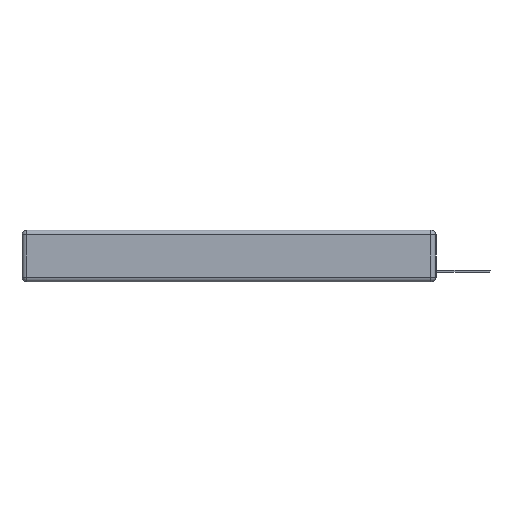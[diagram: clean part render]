
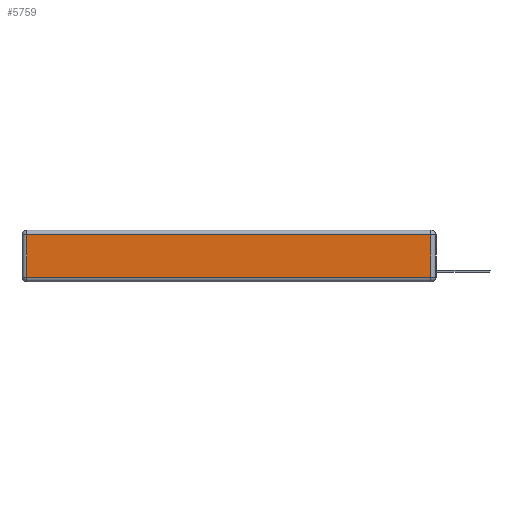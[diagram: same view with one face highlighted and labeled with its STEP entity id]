
A CAD part, left-side view. The second image highlights one B-rep face of the part: STEP entity #5759.
In plain terms, the highlighted planar face has unit normal (-1, 0, 0).
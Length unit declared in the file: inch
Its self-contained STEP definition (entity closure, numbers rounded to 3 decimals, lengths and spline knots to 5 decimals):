
#363 = CARTESIAN_POINT ( 'NONE',  ( 0., 0.03, -0.343 ) ) ;
#465 = EDGE_CURVE ( 'NONE', #4299, #11582, #4855, .T. ) ;
#637 = AXIS2_PLACEMENT_3D ( 'NONE', #4353, #4548, #9961 ) ;
#735 = PLANE ( 'NONE',  #637 ) ;
#736 = ORIENTED_EDGE ( 'NONE', *, *, #11382, .T. ) ;
#1600 = LINE ( 'NONE', #8040, #1606 ) ;
#1606 = VECTOR ( 'NONE', #5298, 39.37008 ) ;
#2235 = LINE ( 'NONE', #363, #11024 ) ;
#2990 = CARTESIAN_POINT ( 'NONE',  ( 0., 0.03, -0.03 ) ) ;
#4062 = EDGE_LOOP ( 'NONE', ( #9951, #736, #7886, #4384 ) ) ;
#4299 = VERTEX_POINT ( 'NONE', #2990 ) ;
#4353 = CARTESIAN_POINT ( 'NONE',  ( 0., 0., -0.343 ) ) ;
#4384 = ORIENTED_EDGE ( 'NONE', *, *, #9934, .T. ) ;
#4548 = DIRECTION ( 'NONE',  ( -1., 0., 0. ) ) ;
#4557 = EDGE_CURVE ( 'NONE', #6209, #8768, #1600, .T. ) ;
#4819 = VECTOR ( 'NONE', #6607, 39.37008 ) ;
#4855 = LINE ( 'NONE', #8523, #7484 ) ;
#5298 = DIRECTION ( 'NONE',  ( 0., -1., 0. ) ) ;
#5411 = CARTESIAN_POINT ( 'NONE',  ( 0., 2.72, -0.313 ) ) ;
#5759 = ADVANCED_FACE ( 'NONE', ( #6425 ), #735, .T. ) ;
#6209 = VERTEX_POINT ( 'NONE', #5411 ) ;
#6425 = FACE_OUTER_BOUND ( 'NONE', #4062, .T. ) ;
#6535 = CARTESIAN_POINT ( 'NONE',  ( 0., 2.72, -0.03 ) ) ;
#6602 = DIRECTION ( 'NONE',  ( 0., 1., 0. ) ) ;
#6607 = DIRECTION ( 'NONE',  ( 0., 0., -1. ) ) ;
#7484 = VECTOR ( 'NONE', #6602, 39.37008 ) ;
#7528 = LINE ( 'NONE', #11335, #4819 ) ;
#7886 = ORIENTED_EDGE ( 'NONE', *, *, #465, .T. ) ;
#8040 = CARTESIAN_POINT ( 'NONE',  ( 0., 0., -0.313 ) ) ;
#8265 = DIRECTION ( 'NONE',  ( 0., 0., 1. ) ) ;
#8523 = CARTESIAN_POINT ( 'NONE',  ( 0., 2.75, -0.03 ) ) ;
#8768 = VERTEX_POINT ( 'NONE', #10067 ) ;
#9934 = EDGE_CURVE ( 'NONE', #11582, #6209, #7528, .T. ) ;
#9951 = ORIENTED_EDGE ( 'NONE', *, *, #4557, .T. ) ;
#9961 = DIRECTION ( 'NONE',  ( 0., 0., 1. ) ) ;
#10067 = CARTESIAN_POINT ( 'NONE',  ( 0., 0.03, -0.313 ) ) ;
#11024 = VECTOR ( 'NONE', #8265, 39.37008 ) ;
#11335 = CARTESIAN_POINT ( 'NONE',  ( 0., 2.72, -0.343 ) ) ;
#11382 = EDGE_CURVE ( 'NONE', #8768, #4299, #2235, .T. ) ;
#11582 = VERTEX_POINT ( 'NONE', #6535 ) ;
